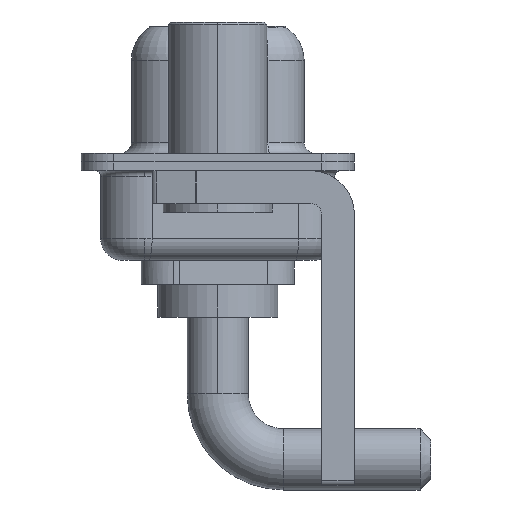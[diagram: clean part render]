
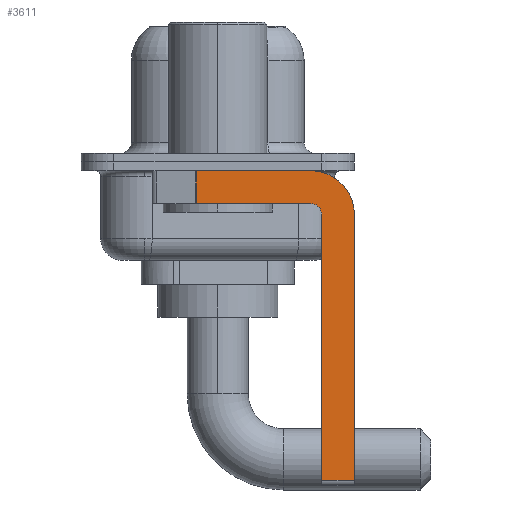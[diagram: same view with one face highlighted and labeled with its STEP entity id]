
A CAD part, left-side view. The second image highlights one B-rep face of the part: STEP entity #3611.
In plain terms, the highlighted planar face has unit normal (-1, 0, 0).
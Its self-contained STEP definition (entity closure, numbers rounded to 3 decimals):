
#121 = DIRECTION ( 'NONE',  ( -1., 0., 0. ) ) ;
#154 = DIRECTION ( 'NONE',  ( 1., 0., 0. ) ) ;
#742 = ORIENTED_EDGE ( 'NONE', *, *, #7947, .F. ) ;
#839 = AXIS2_PLACEMENT_3D ( 'NONE', #13738, #154, #2453 ) ;
#901 = CARTESIAN_POINT ( 'NONE',  ( -2.9, -6.25, -14.55 ) ) ;
#982 = LINE ( 'NONE', #2012, #5452 ) ;
#1051 = ORIENTED_EDGE ( 'NONE', *, *, #1367, .T. ) ;
#1227 = LINE ( 'NONE', #8180, #13784 ) ;
#1367 = EDGE_CURVE ( 'NONE', #14185, #4736, #1227, .T. ) ;
#1562 = CARTESIAN_POINT ( 'NONE',  ( -2.9, -6.25, -2.4 ) ) ;
#1590 = VERTEX_POINT ( 'NONE', #2976 ) ;
#1618 = EDGE_CURVE ( 'NONE', #13188, #8246, #982, .T. ) ;
#1773 = ORIENTED_EDGE ( 'NONE', *, *, #4223, .F. ) ;
#1873 = ORIENTED_EDGE ( 'NONE', *, *, #7854, .F. ) ;
#2012 = CARTESIAN_POINT ( 'NONE',  ( -2.9, -4.25, -1.9 ) ) ;
#2197 = LINE ( 'NONE', #13396, #14274 ) ;
#2438 = DIRECTION ( 'NONE',  ( 0., 0., 1. ) ) ;
#2453 = DIRECTION ( 'NONE',  ( 0., 0., -1. ) ) ;
#2508 = EDGE_CURVE ( 'NONE', #1590, #14286, #6622, .T. ) ;
#2976 = CARTESIAN_POINT ( 'NONE',  ( -2.9, 0.978, -0.4 ) ) ;
#2989 = CIRCLE ( 'NONE', #14373, 0.5 ) ;
#3049 = ORIENTED_EDGE ( 'NONE', *, *, #1618, .F. ) ;
#3156 = DIRECTION ( 'NONE',  ( 0., 0., -1. ) ) ;
#3480 = FACE_OUTER_BOUND ( 'NONE', #7350, .T. ) ;
#3580 = VERTEX_POINT ( 'NONE', #4723 ) ;
#3611 = ADVANCED_FACE ( 'NONE', ( #3480 ), #13585, .F. ) ;
#4155 = ORIENTED_EDGE ( 'NONE', *, *, #4615, .T. ) ;
#4223 = EDGE_CURVE ( 'NONE', #14185, #3580, #8071, .T. ) ;
#4476 = DIRECTION ( 'NONE',  ( 0., -1., 0. ) ) ;
#4615 = EDGE_CURVE ( 'NONE', #1590, #8246, #2197, .T. ) ;
#4723 = CARTESIAN_POINT ( 'NONE',  ( -2.9, -4.75, -2.4 ) ) ;
#4736 = VERTEX_POINT ( 'NONE', #901 ) ;
#5347 = VECTOR ( 'NONE', #2438, 1000. ) ;
#5452 = VECTOR ( 'NONE', #6519, 1000. ) ;
#5813 = DIRECTION ( 'NONE',  ( 0., 0., 1. ) ) ;
#5980 = ORIENTED_EDGE ( 'NONE', *, *, #2508, .F. ) ;
#6064 = AXIS2_PLACEMENT_3D ( 'NONE', #12505, #6255, #9387 ) ;
#6255 = DIRECTION ( 'NONE',  ( 1., 0., 0. ) ) ;
#6519 = DIRECTION ( 'NONE',  ( 0., 1., 0. ) ) ;
#6622 = LINE ( 'NONE', #11156, #9682 ) ;
#6917 = DIRECTION ( 'NONE',  ( 0., -1., 0. ) ) ;
#7350 = EDGE_LOOP ( 'NONE', ( #5980, #4155, #3049, #1873, #1773, #1051, #11641, #742 ) ) ;
#7724 = VECTOR ( 'NONE', #11977, 1000. ) ;
#7727 = CARTESIAN_POINT ( 'NONE',  ( -2.9, -4.25, -0.4 ) ) ;
#7854 = EDGE_CURVE ( 'NONE', #3580, #13188, #2989, .T. ) ;
#7947 = EDGE_CURVE ( 'NONE', #14286, #10478, #14153, .T. ) ;
#7963 = EDGE_CURVE ( 'NONE', #10478, #4736, #14220, .T. ) ;
#8071 = LINE ( 'NONE', #12603, #5347 ) ;
#8180 = CARTESIAN_POINT ( 'NONE',  ( -2.9, -4.25, -14.55 ) ) ;
#8246 = VERTEX_POINT ( 'NONE', #9969 ) ;
#9387 = DIRECTION ( 'NONE',  ( 0., 0., -1. ) ) ;
#9682 = VECTOR ( 'NONE', #4476, 1000. ) ;
#9969 = CARTESIAN_POINT ( 'NONE',  ( -2.9, 0.978, -1.9 ) ) ;
#10478 = VERTEX_POINT ( 'NONE', #1562 ) ;
#10984 = CARTESIAN_POINT ( 'NONE',  ( -2.9, -4.25, -1.9 ) ) ;
#11156 = CARTESIAN_POINT ( 'NONE',  ( -2.9, 3., -0.4 ) ) ;
#11641 = ORIENTED_EDGE ( 'NONE', *, *, #7963, .F. ) ;
#11831 = CARTESIAN_POINT ( 'NONE',  ( -2.9, -6.25, -2.4 ) ) ;
#11977 = DIRECTION ( 'NONE',  ( 0., 0., -1. ) ) ;
#12505 = CARTESIAN_POINT ( 'NONE',  ( -2.9, -4.25, -2.4 ) ) ;
#12603 = CARTESIAN_POINT ( 'NONE',  ( -2.9, -4.75, -14.8 ) ) ;
#13188 = VERTEX_POINT ( 'NONE', #10984 ) ;
#13396 = CARTESIAN_POINT ( 'NONE',  ( -2.9, 0.978, -1.9 ) ) ;
#13585 = PLANE ( 'NONE',  #839 ) ;
#13738 = CARTESIAN_POINT ( 'NONE',  ( -2.9, -4.25, -2.4 ) ) ;
#13780 = CARTESIAN_POINT ( 'NONE',  ( -2.9, -4.25, -2.4 ) ) ;
#13784 = VECTOR ( 'NONE', #6917, 1000. ) ;
#14153 = CIRCLE ( 'NONE', #6064, 2. ) ;
#14185 = VERTEX_POINT ( 'NONE', #14519 ) ;
#14220 = LINE ( 'NONE', #11831, #7724 ) ;
#14274 = VECTOR ( 'NONE', #3156, 1000. ) ;
#14286 = VERTEX_POINT ( 'NONE', #7727 ) ;
#14373 = AXIS2_PLACEMENT_3D ( 'NONE', #13780, #121, #5813 ) ;
#14519 = CARTESIAN_POINT ( 'NONE',  ( -2.9, -4.75, -14.55 ) ) ;
